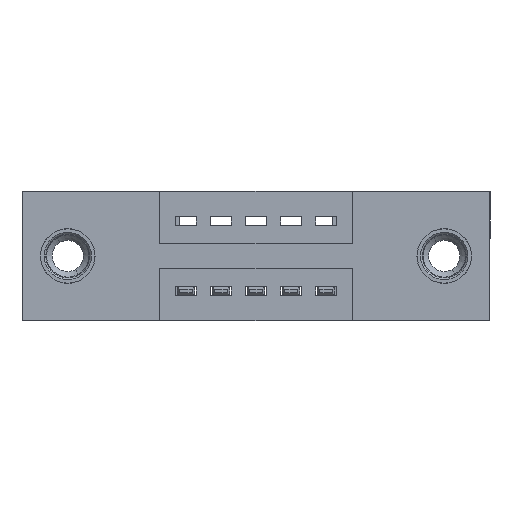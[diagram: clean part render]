
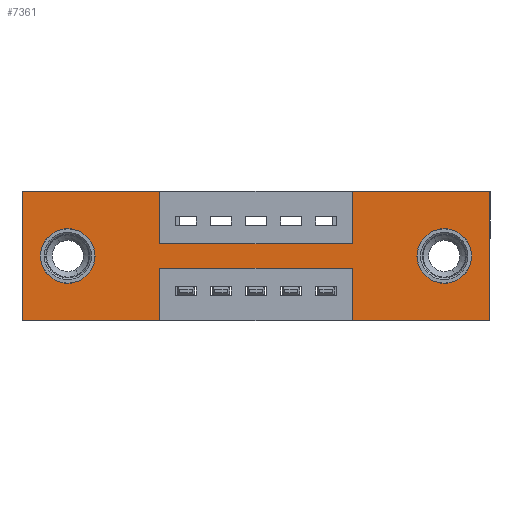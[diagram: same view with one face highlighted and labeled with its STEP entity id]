
A CAD part, front view. The second image highlights one B-rep face of the part: STEP entity #7361.
In plain terms, the highlighted planar face has unit normal (0, -1, 0).
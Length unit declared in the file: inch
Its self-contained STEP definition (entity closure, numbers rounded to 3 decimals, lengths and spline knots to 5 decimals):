
#123 = CARTESIAN_POINT ( 'NONE',  ( 0., 0., 0. ) ) ;
#261 = CARTESIAN_POINT ( 'NONE',  ( 1.335, 0., -0.37 ) ) ;
#300 = VERTEX_POINT ( 'NONE', #5099 ) ;
#329 = CARTESIAN_POINT ( 'NONE',  ( 0.9425, 0., 0. ) ) ;
#453 = VERTEX_POINT ( 'NONE', #6875 ) ;
#523 = CARTESIAN_POINT ( 'NONE',  ( 0.9425, 0., -0.22 ) ) ;
#541 = ORIENTED_EDGE ( 'NONE', *, *, #3352, .F. ) ;
#589 = EDGE_CURVE ( 'NONE', #453, #876, #9067, .T. ) ;
#596 = DIRECTION ( 'NONE',  ( 0., 0., -1. ) ) ;
#645 = EDGE_CURVE ( 'NONE', #677, #3101, #6980, .T. ) ;
#677 = VERTEX_POINT ( 'NONE', #8093 ) ;
#876 = VERTEX_POINT ( 'NONE', #3470 ) ;
#924 = CARTESIAN_POINT ( 'NONE',  ( 0., 0., -0.37 ) ) ;
#942 = AXIS2_PLACEMENT_3D ( 'NONE', #3631, #6094, #10177 ) ;
#949 = CARTESIAN_POINT ( 'NONE',  ( 0.9425, 0., -0.37 ) ) ;
#995 = EDGE_CURVE ( 'NONE', #1690, #300, #8653, .T. ) ;
#1088 = ORIENTED_EDGE ( 'NONE', *, *, #5235, .F. ) ;
#1133 = ORIENTED_EDGE ( 'NONE', *, *, #5925, .F. ) ;
#1138 = AXIS2_PLACEMENT_3D ( 'NONE', #4667, #10453, #596 ) ;
#1169 = ORIENTED_EDGE ( 'NONE', *, *, #9832, .T. ) ;
#1223 = DIRECTION ( 'NONE',  ( 0., 0., -1. ) ) ;
#1247 = DIRECTION ( 'NONE',  ( 1., 0., 0. ) ) ;
#1295 = VECTOR ( 'NONE', #10469, 39.37008 ) ;
#1336 = DIRECTION ( 'NONE',  ( -1., 0., 0. ) ) ;
#1358 = LINE ( 'NONE', #6704, #6505 ) ;
#1501 = CARTESIAN_POINT ( 'NONE',  ( 0.13, 0., -0.185 ) ) ;
#1606 = VERTEX_POINT ( 'NONE', #261 ) ;
#1657 = DIRECTION ( 'NONE',  ( 0., 0., 1. ) ) ;
#1690 = VERTEX_POINT ( 'NONE', #10213 ) ;
#1698 = FACE_BOUND ( 'NONE', #4130, .T. ) ;
#1751 = CARTESIAN_POINT ( 'NONE',  ( 1.335, 0., 0. ) ) ;
#1813 = CARTESIAN_POINT ( 'NONE',  ( 0.9425, 0., -0.37 ) ) ;
#2045 = EDGE_CURVE ( 'NONE', #5542, #6011, #10345, .T. ) ;
#2215 = FACE_OUTER_BOUND ( 'NONE', #10223, .T. ) ;
#2387 = DIRECTION ( 'NONE',  ( 0., 1., 0. ) ) ;
#2538 = ORIENTED_EDGE ( 'NONE', *, *, #8636, .F. ) ;
#2632 = CARTESIAN_POINT ( 'NONE',  ( 0., 0., -0.37 ) ) ;
#2739 = CARTESIAN_POINT ( 'NONE',  ( 1.205, 0., -0.185 ) ) ;
#2859 = VERTEX_POINT ( 'NONE', #6965 ) ;
#2876 = EDGE_LOOP ( 'NONE', ( #1169, #7510 ) ) ;
#3101 = VERTEX_POINT ( 'NONE', #10559 ) ;
#3122 = AXIS2_PLACEMENT_3D ( 'NONE', #1501, #4758, #3127 ) ;
#3127 = DIRECTION ( 'NONE',  ( 0., 0., 1. ) ) ;
#3281 = ORIENTED_EDGE ( 'NONE', *, *, #2045, .F. ) ;
#3352 = EDGE_CURVE ( 'NONE', #6229, #2859, #5643, .T. ) ;
#3458 = VECTOR ( 'NONE', #6740, 39.37008 ) ;
#3468 = AXIS2_PLACEMENT_3D ( 'NONE', #2739, #8510, #9370 ) ;
#3470 = CARTESIAN_POINT ( 'NONE',  ( 0.3925, 0., -0.37 ) ) ;
#3603 = LINE ( 'NONE', #4456, #5776 ) ;
#3631 = CARTESIAN_POINT ( 'NONE',  ( 1.205, 0., -0.185 ) ) ;
#3687 = CARTESIAN_POINT ( 'NONE',  ( 1.335, 0., 0. ) ) ;
#3703 = LINE ( 'NONE', #3687, #9005 ) ;
#3786 = DIRECTION ( 'NONE',  ( 0., 0., -1. ) ) ;
#3862 = CIRCLE ( 'NONE', #942, 0.078 ) ;
#3882 = LINE ( 'NONE', #949, #7116 ) ;
#4130 = EDGE_LOOP ( 'NONE', ( #10258, #9098 ) ) ;
#4296 = DIRECTION ( 'NONE',  ( -1., 0., 0. ) ) ;
#4453 = VECTOR ( 'NONE', #1336, 39.37008 ) ;
#4456 = CARTESIAN_POINT ( 'NONE',  ( 0.3925, 0., 0. ) ) ;
#4504 = EDGE_CURVE ( 'NONE', #1606, #8791, #8079, .T. ) ;
#4667 = CARTESIAN_POINT ( 'NONE',  ( 0., 0., -0.37 ) ) ;
#4682 = VECTOR ( 'NONE', #3786, 39.37008 ) ;
#4687 = DIRECTION ( 'NONE',  ( -1., 0., 0. ) ) ;
#4758 = DIRECTION ( 'NONE',  ( 0., 1., 0. ) ) ;
#5031 = EDGE_CURVE ( 'NONE', #10401, #5656, #6913, .T. ) ;
#5099 = CARTESIAN_POINT ( 'NONE',  ( 1.205, 0., -0.107 ) ) ;
#5197 = ORIENTED_EDGE ( 'NONE', *, *, #6828, .F. ) ;
#5235 = EDGE_CURVE ( 'NONE', #5656, #1606, #3703, .T. ) ;
#5367 = CARTESIAN_POINT ( 'NONE',  ( 0.3925, 0., -0.22 ) ) ;
#5472 = LINE ( 'NONE', #5367, #4453 ) ;
#5542 = VERTEX_POINT ( 'NONE', #8739 ) ;
#5547 = ORIENTED_EDGE ( 'NONE', *, *, #9664, .F. ) ;
#5643 = LINE ( 'NONE', #123, #3458 ) ;
#5656 = VERTEX_POINT ( 'NONE', #1751 ) ;
#5693 = ORIENTED_EDGE ( 'NONE', *, *, #4504, .F. ) ;
#5722 = LINE ( 'NONE', #8936, #9230 ) ;
#5776 = VECTOR ( 'NONE', #1223, 39.37008 ) ;
#5818 = FACE_BOUND ( 'NONE', #2876, .T. ) ;
#5925 = EDGE_CURVE ( 'NONE', #8737, #6229, #1358, .T. ) ;
#6011 = VERTEX_POINT ( 'NONE', #8363 ) ;
#6066 = CARTESIAN_POINT ( 'NONE',  ( 0., 0., 0. ) ) ;
#6094 = DIRECTION ( 'NONE',  ( 0., 1., 0. ) ) ;
#6161 = EDGE_CURVE ( 'NONE', #7369, #453, #5472, .T. ) ;
#6229 = VERTEX_POINT ( 'NONE', #9362 ) ;
#6426 = DIRECTION ( 'NONE',  ( 0., 0., 1. ) ) ;
#6505 = VECTOR ( 'NONE', #1657, 39.37008 ) ;
#6598 = CARTESIAN_POINT ( 'NONE',  ( 0.3925, 0., -0.15 ) ) ;
#6704 = CARTESIAN_POINT ( 'NONE',  ( 0., 0., 0. ) ) ;
#6740 = DIRECTION ( 'NONE',  ( 1., 0., 0. ) ) ;
#6828 = EDGE_CURVE ( 'NONE', #876, #8737, #5722, .T. ) ;
#6875 = CARTESIAN_POINT ( 'NONE',  ( 0.3925, 0., -0.22 ) ) ;
#6913 = LINE ( 'NONE', #6066, #8593 ) ;
#6965 = CARTESIAN_POINT ( 'NONE',  ( 0.3925, 0., 0. ) ) ;
#6972 = LINE ( 'NONE', #329, #1295 ) ;
#6980 = CIRCLE ( 'NONE', #3122, 0.078 ) ;
#7116 = VECTOR ( 'NONE', #9915, 39.37008 ) ;
#7246 = CARTESIAN_POINT ( 'NONE',  ( 0.13, 0., -0.185 ) ) ;
#7334 = CIRCLE ( 'NONE', #8757, 0.078 ) ;
#7361 = ADVANCED_FACE ( 'NONE', ( #5818, #1698, #2215 ), #7940, .T. ) ;
#7369 = VERTEX_POINT ( 'NONE', #523 ) ;
#7510 = ORIENTED_EDGE ( 'NONE', *, *, #995, .T. ) ;
#7823 = CARTESIAN_POINT ( 'NONE',  ( 0.3925, 0., -0.37 ) ) ;
#7940 = PLANE ( 'NONE',  #1138 ) ;
#8079 = LINE ( 'NONE', #2632, #9541 ) ;
#8093 = CARTESIAN_POINT ( 'NONE',  ( 0.13, 0., -0.263 ) ) ;
#8363 = CARTESIAN_POINT ( 'NONE',  ( 0.9425, 0., -0.15 ) ) ;
#8510 = DIRECTION ( 'NONE',  ( 0., 1., 0. ) ) ;
#8593 = VECTOR ( 'NONE', #1247, 39.37008 ) ;
#8611 = EDGE_CURVE ( 'NONE', #8791, #7369, #3882, .T. ) ;
#8636 = EDGE_CURVE ( 'NONE', #6011, #10401, #6972, .T. ) ;
#8652 = CARTESIAN_POINT ( 'NONE',  ( 0.9425, 0., 0. ) ) ;
#8653 = CIRCLE ( 'NONE', #3468, 0.078 ) ;
#8670 = DIRECTION ( 'NONE',  ( 0., 0., -1. ) ) ;
#8737 = VERTEX_POINT ( 'NONE', #924 ) ;
#8739 = CARTESIAN_POINT ( 'NONE',  ( 0.3925, 0., -0.15 ) ) ;
#8757 = AXIS2_PLACEMENT_3D ( 'NONE', #7246, #2387, #6426 ) ;
#8791 = VERTEX_POINT ( 'NONE', #1813 ) ;
#8936 = CARTESIAN_POINT ( 'NONE',  ( 0., 0., -0.37 ) ) ;
#9004 = ORIENTED_EDGE ( 'NONE', *, *, #8611, .F. ) ;
#9005 = VECTOR ( 'NONE', #8670, 39.37008 ) ;
#9067 = LINE ( 'NONE', #7823, #4682 ) ;
#9098 = ORIENTED_EDGE ( 'NONE', *, *, #645, .T. ) ;
#9159 = ORIENTED_EDGE ( 'NONE', *, *, #5031, .F. ) ;
#9230 = VECTOR ( 'NONE', #4687, 39.37008 ) ;
#9362 = CARTESIAN_POINT ( 'NONE',  ( 0., 0., 0. ) ) ;
#9370 = DIRECTION ( 'NONE',  ( 0., 0., -1. ) ) ;
#9541 = VECTOR ( 'NONE', #4296, 39.37008 ) ;
#9664 = EDGE_CURVE ( 'NONE', #2859, #5542, #3603, .T. ) ;
#9737 = ORIENTED_EDGE ( 'NONE', *, *, #6161, .F. ) ;
#9832 = EDGE_CURVE ( 'NONE', #300, #1690, #3862, .T. ) ;
#9879 = ORIENTED_EDGE ( 'NONE', *, *, #589, .F. ) ;
#9915 = DIRECTION ( 'NONE',  ( 0., 0., 1. ) ) ;
#9964 = DIRECTION ( 'NONE',  ( 1., 0., 0. ) ) ;
#10177 = DIRECTION ( 'NONE',  ( 0., 0., -1. ) ) ;
#10208 = VECTOR ( 'NONE', #9964, 39.37008 ) ;
#10213 = CARTESIAN_POINT ( 'NONE',  ( 1.205, 0., -0.263 ) ) ;
#10223 = EDGE_LOOP ( 'NONE', ( #9879, #9737, #9004, #5693, #1088, #9159, #2538, #3281, #5547, #541, #1133, #5197 ) ) ;
#10258 = ORIENTED_EDGE ( 'NONE', *, *, #10534, .T. ) ;
#10345 = LINE ( 'NONE', #6598, #10208 ) ;
#10401 = VERTEX_POINT ( 'NONE', #8652 ) ;
#10453 = DIRECTION ( 'NONE',  ( 0., -1., 0. ) ) ;
#10469 = DIRECTION ( 'NONE',  ( 0., 0., 1. ) ) ;
#10534 = EDGE_CURVE ( 'NONE', #3101, #677, #7334, .T. ) ;
#10559 = CARTESIAN_POINT ( 'NONE',  ( 0.13, 0., -0.107 ) ) ;
